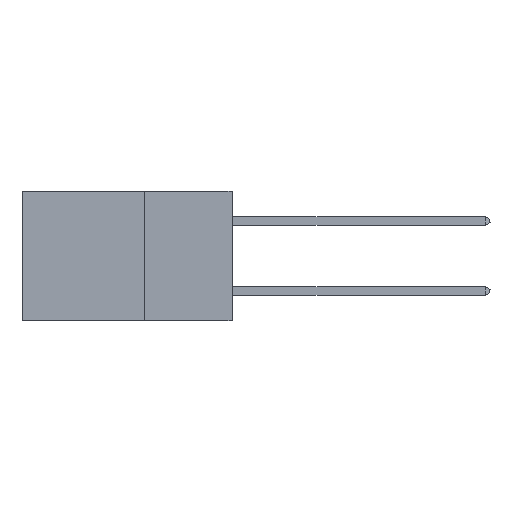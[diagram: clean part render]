
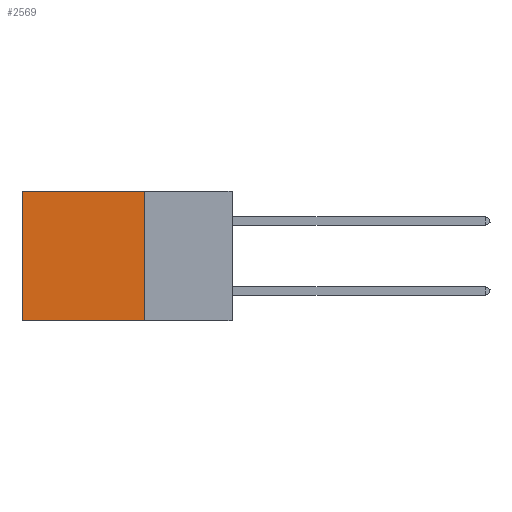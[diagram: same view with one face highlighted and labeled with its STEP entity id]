
A CAD part, left-side view. The second image highlights one B-rep face of the part: STEP entity #2569.
In plain terms, the highlighted planar face has unit normal (-1, 0, 0).
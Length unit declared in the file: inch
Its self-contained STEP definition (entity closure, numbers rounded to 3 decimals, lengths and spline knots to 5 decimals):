
#2569 = ADVANCED_FACE ( 'NONE', ( #24988 ), #25474, .F. ) ;
#5636 = ORIENTED_EDGE ( 'NONE', *, *, #6825, .F. ) ;
#5797 = AXIS2_PLACEMENT_3D ( 'NONE', #14389, #12868, #34752 ) ;
#6428 = DIRECTION ( 'NONE',  ( 0., 1., 0. ) ) ;
#6825 = EDGE_CURVE ( 'NONE', #37683, #16752, #39331, .T. ) ;
#7060 = VECTOR ( 'NONE', #32736, 39.37008 ) ;
#10678 = VERTEX_POINT ( 'NONE', #27749 ) ;
#10792 = CARTESIAN_POINT ( 'NONE',  ( 0.2875, 0.25, 0. ) ) ;
#12384 = CARTESIAN_POINT ( 'NONE',  ( 0.2875, 0.25, -0.37 ) ) ;
#12868 = DIRECTION ( 'NONE',  ( 1., 0., 0. ) ) ;
#13352 = EDGE_LOOP ( 'NONE', ( #28915, #30525, #5636, #31935 ) ) ;
#14248 = VECTOR ( 'NONE', #23872, 39.37008 ) ;
#14389 = CARTESIAN_POINT ( 'NONE',  ( 0.2875, 0.25, 0. ) ) ;
#16752 = VERTEX_POINT ( 'NONE', #12384 ) ;
#17325 = VECTOR ( 'NONE', #6428, 39.37008 ) ;
#18331 = LINE ( 'NONE', #22312, #17325 ) ;
#20039 = LINE ( 'NONE', #21037, #29248 ) ;
#21037 = CARTESIAN_POINT ( 'NONE',  ( 0.2875, 0.25, 0. ) ) ;
#22312 = CARTESIAN_POINT ( 'NONE',  ( 0.2875, 0.25, -0.37 ) ) ;
#22534 = EDGE_CURVE ( 'NONE', #37683, #10678, #20039, .T. ) ;
#22676 = LINE ( 'NONE', #29954, #14248 ) ;
#23872 = DIRECTION ( 'NONE',  ( 0., 0., -1. ) ) ;
#23969 = CARTESIAN_POINT ( 'NONE',  ( 0.2875, 0.25, 0. ) ) ;
#24988 = FACE_OUTER_BOUND ( 'NONE', #13352, .T. ) ;
#25474 = PLANE ( 'NONE',  #5797 ) ;
#27749 = CARTESIAN_POINT ( 'NONE',  ( 0.2875, 0.6, 0. ) ) ;
#28915 = ORIENTED_EDGE ( 'NONE', *, *, #29094, .T. ) ;
#29094 = EDGE_CURVE ( 'NONE', #10678, #36871, #22676, .T. ) ;
#29248 = VECTOR ( 'NONE', #36530, 39.37008 ) ;
#29954 = CARTESIAN_POINT ( 'NONE',  ( 0.2875, 0.6, 0. ) ) ;
#30525 = ORIENTED_EDGE ( 'NONE', *, *, #38014, .F. ) ;
#31935 = ORIENTED_EDGE ( 'NONE', *, *, #22534, .T. ) ;
#32736 = DIRECTION ( 'NONE',  ( 0., 0., -1. ) ) ;
#34752 = DIRECTION ( 'NONE',  ( 0., 0., -1. ) ) ;
#36530 = DIRECTION ( 'NONE',  ( 0., 1., 0. ) ) ;
#36871 = VERTEX_POINT ( 'NONE', #37988 ) ;
#37683 = VERTEX_POINT ( 'NONE', #23969 ) ;
#37988 = CARTESIAN_POINT ( 'NONE',  ( 0.2875, 0.6, -0.37 ) ) ;
#38014 = EDGE_CURVE ( 'NONE', #16752, #36871, #18331, .T. ) ;
#39331 = LINE ( 'NONE', #10792, #7060 ) ;
